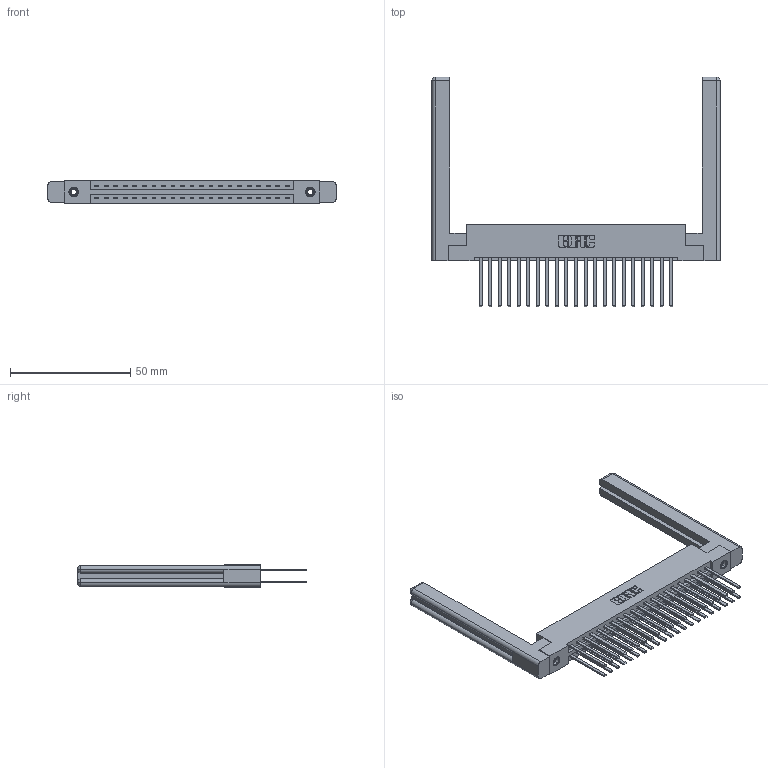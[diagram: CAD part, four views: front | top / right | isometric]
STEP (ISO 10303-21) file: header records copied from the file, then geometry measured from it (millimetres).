
FILE_DESCRIPTION (( 'STEP AP203' ), '1' );
FILE_NAME ('387-042-544-258.STEP', '2019-10-18T04:23:09', ( '' ), ( '' ), 'SwSTEP 2.0', 'SolidWorks 2016', '' );
FILE_SCHEMA (( 'CONFIG_CONTROL_DESIGN' ));
Length unit declared in the file: inch
Products named in the file (5): 345-292-001_345-293-144; 307-220-058; 345-250-001_345-250-001-102; 337 Part_Flush Mounting Lugs - 0.156 Dia-TI; 387-042-544-258
Assembly tree (47 placements, depth 2):
  387-042-544-258
    337 Part_Flush Mounting Lugs - 0.156 Dia-TI
    345-292-001_345-293-144  x42
    345-250-001_345-250-001-102  x2
    307-220-058  x2
Bounding box: 119.84 x 95.38 x 9.4 mm (x, y, z)
Volume: 20081 mm3; surface area: 21393.2 mm2
Topology: 47 solids, 47 shells, 2272 faces, 6671 edges, 4378 vertices
Faces by surface type: plane 1582, cylinder 666, cone 12, torus 12
Entity records: 21448 total; most frequent: CARTESIAN_POINT 3637, ORIENTED_EDGE 3512, DIRECTION 3144, EDGE_CURVE 1756, VECTOR 1584, LINE 1584, VERTEX_POINT 1162, AXIS2_PLACEMENT_3D 780
